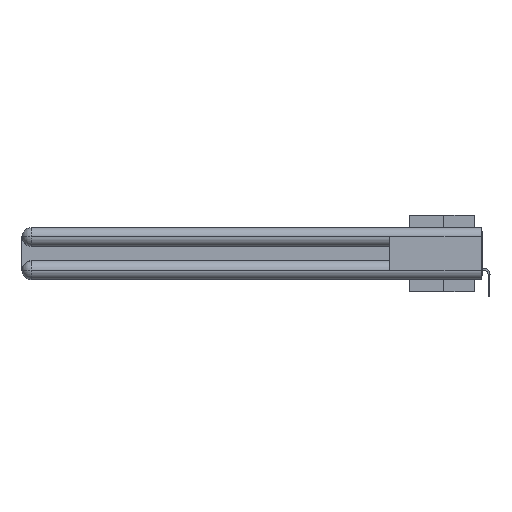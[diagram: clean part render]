
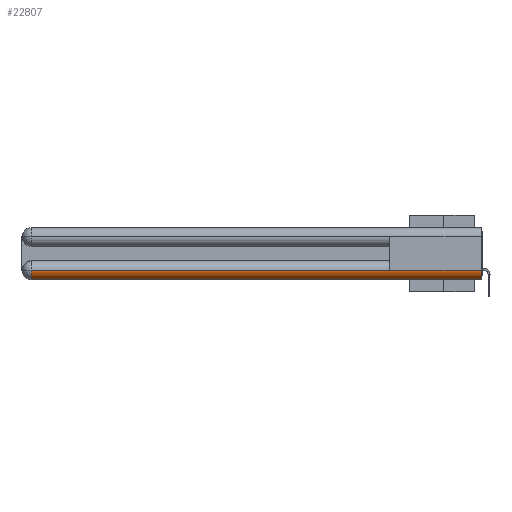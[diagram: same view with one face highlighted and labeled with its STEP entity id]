
A CAD part, left-side view. The second image highlights one B-rep face of the part: STEP entity #22807.
In plain terms, the highlighted cylindrical face has radius 1.562 mm (diameter 3.124 mm), a partial arc.
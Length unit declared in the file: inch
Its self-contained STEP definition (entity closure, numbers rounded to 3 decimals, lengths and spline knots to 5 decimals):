
#1468 = VECTOR ( 'NONE', #33641, 39.37008 ) ;
#2105 = CARTESIAN_POINT ( 'NONE',  ( 0.0615, 0., -0.34 ) ) ;
#2725 = LINE ( 'NONE', #34021, #38809 ) ;
#4068 = DIRECTION ( 'NONE',  ( 0., 0., -1. ) ) ;
#4457 = VERTEX_POINT ( 'NONE', #2105 ) ;
#4460 = FACE_OUTER_BOUND ( 'NONE', #37042, .T. ) ;
#5667 = DIRECTION ( 'NONE',  ( 0., -1., 0. ) ) ;
#5944 = EDGE_CURVE ( 'NONE', #19889, #4457, #36600, .T. ) ;
#6534 = CARTESIAN_POINT ( 'NONE',  ( 0.0615, 2.94, -0.34 ) ) ;
#7067 = EDGE_CURVE ( 'NONE', #34121, #19889, #2725, .T. ) ;
#8272 = ORIENTED_EDGE ( 'NONE', *, *, #18332, .T. ) ;
#9339 = ORIENTED_EDGE ( 'NONE', *, *, #9968, .T. ) ;
#9968 = EDGE_CURVE ( 'NONE', #24882, #13352, #16504, .T. ) ;
#10171 = DIRECTION ( 'NONE',  ( 0., -1., 0. ) ) ;
#12073 = CARTESIAN_POINT ( 'NONE',  ( 0., 0., -0.2785 ) ) ;
#12171 = ORIENTED_EDGE ( 'NONE', *, *, #5944, .F. ) ;
#13352 = VERTEX_POINT ( 'NONE', #6534 ) ;
#13986 = VECTOR ( 'NONE', #33580, 39.37008 ) ;
#15817 = EDGE_CURVE ( 'NONE', #4457, #13352, #30688, .T. ) ;
#16504 = CIRCLE ( 'NONE', #30673, 0.0615 ) ;
#17115 = CARTESIAN_POINT ( 'NONE',  ( 0.0615, 0., -0.2785 ) ) ;
#18332 = EDGE_CURVE ( 'NONE', #34121, #24882, #30535, .T. ) ;
#19042 = ORIENTED_EDGE ( 'NONE', *, *, #15817, .F. ) ;
#19281 = CARTESIAN_POINT ( 'NONE',  ( 0.0615, 2.94, -0.2785 ) ) ;
#19889 = VERTEX_POINT ( 'NONE', #12073 ) ;
#21935 = DIRECTION ( 'NONE',  ( 0., -1., 0. ) ) ;
#22807 = ADVANCED_FACE ( 'NONE', ( #4460 ), #26011, .T. ) ;
#23708 = CARTESIAN_POINT ( 'NONE',  ( 0., 0., -0.2785 ) ) ;
#24882 = VERTEX_POINT ( 'NONE', #29014 ) ;
#26011 = CYLINDRICAL_SURFACE ( 'NONE', #27703, 0.0615 ) ;
#27354 = CARTESIAN_POINT ( 'NONE',  ( 0.0615, 0., -0.2785 ) ) ;
#27703 = AXIS2_PLACEMENT_3D ( 'NONE', #17115, #29326, #4068 ) ;
#28151 = DIRECTION ( 'NONE',  ( 1., 0., 0. ) ) ;
#29014 = CARTESIAN_POINT ( 'NONE',  ( 0., 2.94, -0.2785 ) ) ;
#29326 = DIRECTION ( 'NONE',  ( 0., -1., 0. ) ) ;
#30535 = LINE ( 'NONE', #23708, #1468 ) ;
#30673 = AXIS2_PLACEMENT_3D ( 'NONE', #19281, #10171, #34822 ) ;
#30688 = LINE ( 'NONE', #40218, #13986 ) ;
#32253 = ORIENTED_EDGE ( 'NONE', *, *, #7067, .F. ) ;
#33580 = DIRECTION ( 'NONE',  ( 0., 1., 0. ) ) ;
#33641 = DIRECTION ( 'NONE',  ( 0., 1., 0. ) ) ;
#34021 = CARTESIAN_POINT ( 'NONE',  ( 0., 0., -0.2785 ) ) ;
#34121 = VERTEX_POINT ( 'NONE', #40165 ) ;
#34822 = DIRECTION ( 'NONE',  ( 0., 0., 1. ) ) ;
#36600 = CIRCLE ( 'NONE', #37923, 0.0615 ) ;
#37042 = EDGE_LOOP ( 'NONE', ( #8272, #9339, #19042, #12171, #32253 ) ) ;
#37923 = AXIS2_PLACEMENT_3D ( 'NONE', #27354, #21935, #28151 ) ;
#38809 = VECTOR ( 'NONE', #5667, 39.37008 ) ;
#40165 = CARTESIAN_POINT ( 'NONE',  ( 0., 0.6, -0.2785 ) ) ;
#40218 = CARTESIAN_POINT ( 'NONE',  ( 0.0615, 0., -0.34 ) ) ;
